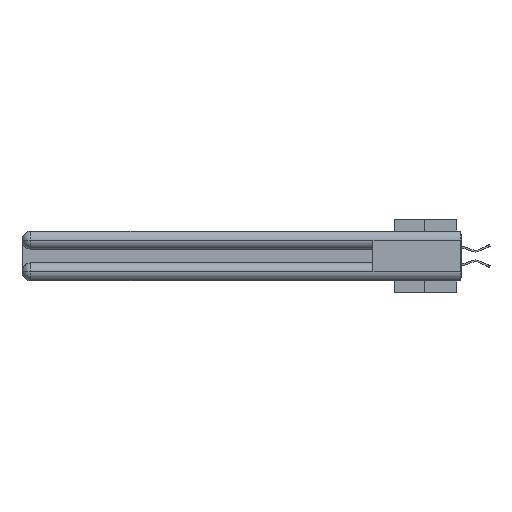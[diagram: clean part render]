
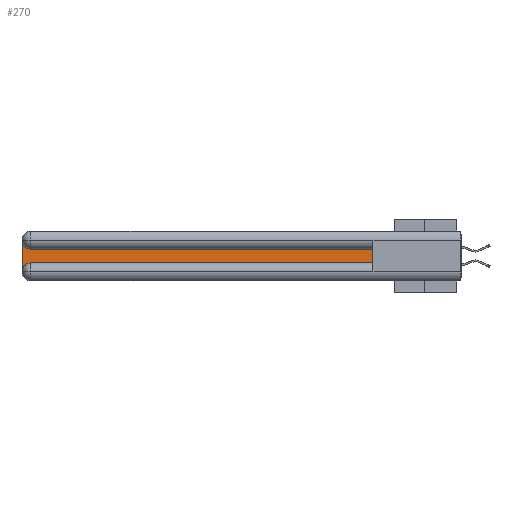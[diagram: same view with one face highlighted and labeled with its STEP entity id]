
A CAD part, left-side view. The second image highlights one B-rep face of the part: STEP entity #270.
In plain terms, the highlighted planar face has unit normal (-1, 0, 0).
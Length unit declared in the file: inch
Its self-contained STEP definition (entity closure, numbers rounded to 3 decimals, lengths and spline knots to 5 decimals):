
#270 = ADVANCED_FACE ( 'NONE', ( #35962 ), #842, .F. ) ;
#672 = EDGE_CURVE ( 'NONE', #7515, #9966, #36375, .T. ) ;
#842 = PLANE ( 'NONE',  #25803 ) ;
#1277 = VECTOR ( 'NONE', #25357, 39.37008 ) ;
#1293 = VECTOR ( 'NONE', #6104, 39.37008 ) ;
#1556 = CIRCLE ( 'NONE', #16606, 0.06 ) ;
#2767 = DIRECTION ( 'NONE',  ( 1., 0., 0. ) ) ;
#3377 = ORIENTED_EDGE ( 'NONE', *, *, #37131, .T. ) ;
#4164 = VECTOR ( 'NONE', #10139, 39.37008 ) ;
#4520 = VERTEX_POINT ( 'NONE', #5683 ) ;
#5281 = DIRECTION ( 'NONE',  ( 0., 0., -1. ) ) ;
#5481 = ORIENTED_EDGE ( 'NONE', *, *, #38574, .T. ) ;
#5683 = CARTESIAN_POINT ( 'NONE',  ( 0.075, 3., -0.0625 ) ) ;
#5733 = EDGE_CURVE ( 'NONE', #4520, #34124, #6438, .T. ) ;
#6104 = DIRECTION ( 'NONE',  ( 0., 0., -1. ) ) ;
#6438 = LINE ( 'NONE', #12046, #1293 ) ;
#7122 = CARTESIAN_POINT ( 'NONE',  ( 0.075, 0.6, -0.2175 ) ) ;
#7515 = VERTEX_POINT ( 'NONE', #7122 ) ;
#9335 = EDGE_LOOP ( 'NONE', ( #20686, #30459, #23439, #3377, #5481, #28930 ) ) ;
#9849 = CARTESIAN_POINT ( 'NONE',  ( 0.075, 3., -0.1225 ) ) ;
#9966 = VERTEX_POINT ( 'NONE', #12910 ) ;
#10139 = DIRECTION ( 'NONE',  ( 0., 1., 0. ) ) ;
#12046 = CARTESIAN_POINT ( 'NONE',  ( 0.075, 3., -0.2175 ) ) ;
#12523 = DIRECTION ( 'NONE',  ( 0., 0., 1. ) ) ;
#12910 = CARTESIAN_POINT ( 'NONE',  ( 0.075, 0.6, -0.1225 ) ) ;
#14365 = VECTOR ( 'NONE', #12523, 39.37008 ) ;
#14589 = CARTESIAN_POINT ( 'NONE',  ( 0.075, 3., -0.2775 ) ) ;
#15843 = DIRECTION ( 'NONE',  ( 1., 0., 0. ) ) ;
#15951 = CARTESIAN_POINT ( 'NONE',  ( 0.075, 2.94, -0.1225 ) ) ;
#16606 = AXIS2_PLACEMENT_3D ( 'NONE', #17788, #2767, #5281 ) ;
#17137 = LINE ( 'NONE', #22242, #1277 ) ;
#17788 = CARTESIAN_POINT ( 'NONE',  ( 0.075, 2.94, -0.2775 ) ) ;
#18293 = CARTESIAN_POINT ( 'NONE',  ( 0.075, 2.94, -0.2175 ) ) ;
#20441 = EDGE_CURVE ( 'NONE', #9966, #21164, #31313, .T. ) ;
#20502 = EDGE_CURVE ( 'NONE', #21164, #4520, #22182, .T. ) ;
#20686 = ORIENTED_EDGE ( 'NONE', *, *, #20441, .T. ) ;
#21164 = VERTEX_POINT ( 'NONE', #15951 ) ;
#21666 = CARTESIAN_POINT ( 'NONE',  ( 0.075, 0.6, -0.1225 ) ) ;
#22182 = CIRCLE ( 'NONE', #36707, 0.06 ) ;
#22195 = DIRECTION ( 'NONE',  ( 0., 0., -1. ) ) ;
#22204 = VERTEX_POINT ( 'NONE', #18293 ) ;
#22242 = CARTESIAN_POINT ( 'NONE',  ( 0.075, 0.6, -0.2175 ) ) ;
#23439 = ORIENTED_EDGE ( 'NONE', *, *, #5733, .T. ) ;
#24808 = CARTESIAN_POINT ( 'NONE',  ( 0.075, 2.94, -0.0625 ) ) ;
#25357 = DIRECTION ( 'NONE',  ( 0., -1., 0. ) ) ;
#25803 = AXIS2_PLACEMENT_3D ( 'NONE', #9849, #15843, #36790 ) ;
#28930 = ORIENTED_EDGE ( 'NONE', *, *, #672, .T. ) ;
#30459 = ORIENTED_EDGE ( 'NONE', *, *, #20502, .T. ) ;
#30507 = CARTESIAN_POINT ( 'NONE',  ( 0.075, 0.6, -0.2175 ) ) ;
#31313 = LINE ( 'NONE', #21666, #4164 ) ;
#33692 = DIRECTION ( 'NONE',  ( 1., 0., 0. ) ) ;
#34124 = VERTEX_POINT ( 'NONE', #14589 ) ;
#35962 = FACE_OUTER_BOUND ( 'NONE', #9335, .T. ) ;
#36375 = LINE ( 'NONE', #30507, #14365 ) ;
#36707 = AXIS2_PLACEMENT_3D ( 'NONE', #24808, #33692, #22195 ) ;
#36790 = DIRECTION ( 'NONE',  ( 0., 0., -1. ) ) ;
#37131 = EDGE_CURVE ( 'NONE', #34124, #22204, #1556, .T. ) ;
#38574 = EDGE_CURVE ( 'NONE', #22204, #7515, #17137, .T. ) ;
